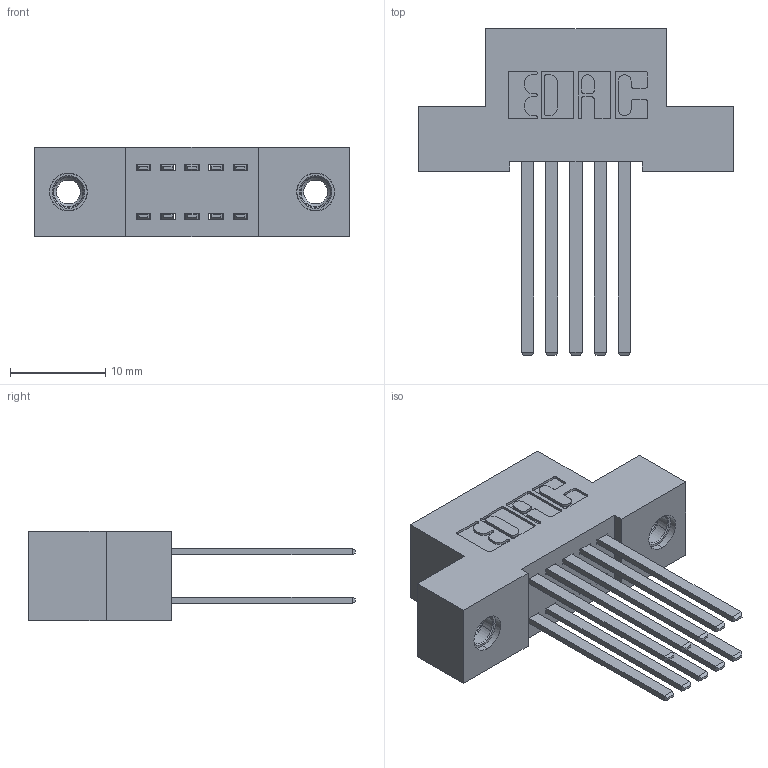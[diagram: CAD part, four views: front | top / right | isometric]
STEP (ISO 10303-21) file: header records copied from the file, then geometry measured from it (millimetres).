
FILE_DESCRIPTION (( 'STEP AP203' ), '1' );
FILE_NAME ('392-010-544-207.STEP', '2019-10-05T01:06:18', ( '' ), ( '' ), 'SwSTEP 2.0', 'SolidWorks 2016', '' );
FILE_SCHEMA (( 'CONFIG_CONTROL_DESIGN' ));
Length unit declared in the file: inch
Products named in the file (4): 345-292-001_345-293-144; 345-250-001_345-250-005-103; 392-010-544-207; 342 Part_TI
Assembly tree (13 placements, depth 2):
  392-010-544-207
    342 Part_TI
    345-292-001_345-293-144  x10
    345-250-001_345-250-005-103  x2
Bounding box: 33.02 x 34.3 x 9.4 mm (x, y, z)
Volume: 2919.2 mm3; surface area: 4254 mm2
Topology: 13 solids, 13 shells, 630 faces, 1805 edges, 1182 vertices
Faces by surface type: plane 418, cylinder 196, cone 12, torus 4
Entity records: 8872 total; most frequent: CARTESIAN_POINT 1493, ORIENTED_EDGE 1422, DIRECTION 1369, EDGE_CURVE 711, LINE 567, VECTOR 567, VERTEX_POINT 468, AXIS2_PLACEMENT_3D 401
